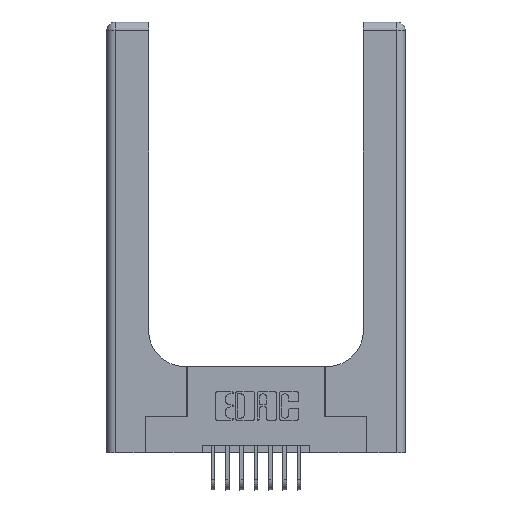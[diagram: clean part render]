
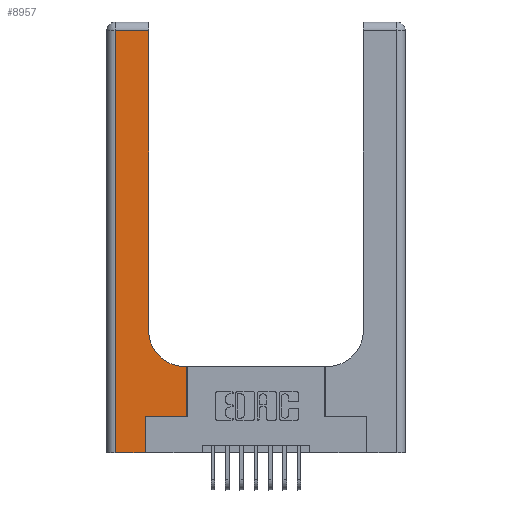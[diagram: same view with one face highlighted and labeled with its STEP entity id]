
A CAD part, top view. The second image highlights one B-rep face of the part: STEP entity #8957.
In plain terms, the highlighted planar face has unit normal (0, 0, 1).
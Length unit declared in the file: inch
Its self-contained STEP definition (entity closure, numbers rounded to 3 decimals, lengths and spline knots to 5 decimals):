
#99 = ORIENTED_EDGE ( 'NONE', *, *, #4465, .T. ) ;
#174 = LINE ( 'NONE', #6906, #6595 ) ;
#306 = AXIS2_PLACEMENT_3D ( 'NONE', #1121, #5297, #14372 ) ;
#1121 = CARTESIAN_POINT ( 'NONE',  ( 0., 3., 0.37 ) ) ;
#1159 = ORIENTED_EDGE ( 'NONE', *, *, #1406, .T. ) ;
#1214 = ORIENTED_EDGE ( 'NONE', *, *, #3346, .T. ) ;
#1329 = ORIENTED_EDGE ( 'NONE', *, *, #3376, .T. ) ;
#1394 = VERTEX_POINT ( 'NONE', #12802 ) ;
#1406 = EDGE_CURVE ( 'NONE', #1394, #3096, #4149, .T. ) ;
#1425 = VERTEX_POINT ( 'NONE', #12467 ) ;
#1510 = LINE ( 'NONE', #16889, #15101 ) ;
#1581 = ORIENTED_EDGE ( 'NONE', *, *, #5345, .T. ) ;
#1689 = VECTOR ( 'NONE', #13584, 39.37008 ) ;
#2341 = CIRCLE ( 'NONE', #14612, 0.25 ) ;
#2846 = DIRECTION ( 'NONE',  ( 0., 0., -1. ) ) ;
#3096 = VERTEX_POINT ( 'NONE', #14969 ) ;
#3267 = CARTESIAN_POINT ( 'NONE',  ( 0.5415, 0.6, 0.37 ) ) ;
#3346 = EDGE_CURVE ( 'NONE', #13283, #1394, #9100, .T. ) ;
#3376 = EDGE_CURVE ( 'NONE', #1425, #16969, #1510, .T. ) ;
#3851 = DIRECTION ( 'NONE',  ( 0., -1., 0. ) ) ;
#3909 = VERTEX_POINT ( 'NONE', #16985 ) ;
#4041 = EDGE_CURVE ( 'NONE', #3096, #5231, #174, .T. ) ;
#4146 = EDGE_CURVE ( 'NONE', #5231, #3909, #4934, .T. ) ;
#4149 = LINE ( 'NONE', #12658, #13765 ) ;
#4465 = EDGE_CURVE ( 'NONE', #16969, #13283, #8037, .T. ) ;
#4934 = LINE ( 'NONE', #12531, #15663 ) ;
#5231 = VERTEX_POINT ( 'NONE', #8025 ) ;
#5243 = ORIENTED_EDGE ( 'NONE', *, *, #4146, .T. ) ;
#5297 = DIRECTION ( 'NONE',  ( 0., 0., -1. ) ) ;
#5345 = EDGE_CURVE ( 'NONE', #3909, #15047, #5358, .T. ) ;
#5357 = DIRECTION ( 'NONE',  ( 0., 1., 0. ) ) ;
#5358 = LINE ( 'NONE', #16061, #1689 ) ;
#5701 = ORIENTED_EDGE ( 'NONE', *, *, #11182, .T. ) ;
#5800 = DIRECTION ( 'NONE',  ( -1., 0., 0. ) ) ;
#6087 = ORIENTED_EDGE ( 'NONE', *, *, #4041, .T. ) ;
#6595 = VECTOR ( 'NONE', #15938, 39.37008 ) ;
#6906 = CARTESIAN_POINT ( 'NONE',  ( 0.269, 0., 0.37 ) ) ;
#7867 = CARTESIAN_POINT ( 'NONE',  ( 0., 2.94, 0.37 ) ) ;
#8025 = CARTESIAN_POINT ( 'NONE',  ( 0.269, 0.25, 0.37 ) ) ;
#8037 = LINE ( 'NONE', #7867, #14897 ) ;
#8122 = EDGE_LOOP ( 'NONE', ( #1329, #99, #1214, #1159, #6087, #5243, #1581, #5701, #9970 ) ) ;
#8163 = LINE ( 'NONE', #9796, #14629 ) ;
#8587 = DIRECTION ( 'NONE',  ( 1., 0., 0. ) ) ;
#8628 = CARTESIAN_POINT ( 'NONE',  ( 0.2915, 2.94, 0.37 ) ) ;
#8957 = ADVANCED_FACE ( 'NONE', ( #16131 ), #11827, .F. ) ;
#9100 = LINE ( 'NONE', #13112, #15888 ) ;
#9796 = CARTESIAN_POINT ( 'NONE',  ( 0.2915, 0.6, 0.37 ) ) ;
#9944 = CARTESIAN_POINT ( 'NONE',  ( 0.06, 2.94, 0.37 ) ) ;
#9970 = ORIENTED_EDGE ( 'NONE', *, *, #16236, .T. ) ;
#10869 = CARTESIAN_POINT ( 'NONE',  ( 0.5415, 0.85, 0.37 ) ) ;
#11182 = EDGE_CURVE ( 'NONE', #15047, #13286, #8163, .T. ) ;
#11827 = PLANE ( 'NONE',  #306 ) ;
#12141 = DIRECTION ( 'NONE',  ( 1., 0., 0. ) ) ;
#12467 = CARTESIAN_POINT ( 'NONE',  ( 0.2915, 0.85, 0.37 ) ) ;
#12531 = CARTESIAN_POINT ( 'NONE',  ( 0.269, 0.25, 0.37 ) ) ;
#12572 = DIRECTION ( 'NONE',  ( 1., 0., 0. ) ) ;
#12658 = CARTESIAN_POINT ( 'NONE',  ( 0., 0., 0.37 ) ) ;
#12802 = CARTESIAN_POINT ( 'NONE',  ( 0.06, 0., 0.37 ) ) ;
#13112 = CARTESIAN_POINT ( 'NONE',  ( 0.06, 3., 0.37 ) ) ;
#13283 = VERTEX_POINT ( 'NONE', #9944 ) ;
#13286 = VERTEX_POINT ( 'NONE', #3267 ) ;
#13584 = DIRECTION ( 'NONE',  ( 0., 1., 0. ) ) ;
#13765 = VECTOR ( 'NONE', #12572, 39.37008 ) ;
#14372 = DIRECTION ( 'NONE',  ( -1., 0., 0. ) ) ;
#14612 = AXIS2_PLACEMENT_3D ( 'NONE', #10869, #2846, #12141 ) ;
#14629 = VECTOR ( 'NONE', #5800, 39.37008 ) ;
#14897 = VECTOR ( 'NONE', #16853, 39.37008 ) ;
#14969 = CARTESIAN_POINT ( 'NONE',  ( 0.269, 0., 0.37 ) ) ;
#15047 = VERTEX_POINT ( 'NONE', #16176 ) ;
#15101 = VECTOR ( 'NONE', #5357, 39.37008 ) ;
#15663 = VECTOR ( 'NONE', #8587, 39.37008 ) ;
#15888 = VECTOR ( 'NONE', #3851, 39.37008 ) ;
#15938 = DIRECTION ( 'NONE',  ( 0., 1., 0. ) ) ;
#16061 = CARTESIAN_POINT ( 'NONE',  ( 0.5585, 0.25, 0.37 ) ) ;
#16131 = FACE_OUTER_BOUND ( 'NONE', #8122, .T. ) ;
#16176 = CARTESIAN_POINT ( 'NONE',  ( 0.5585, 0.6, 0.37 ) ) ;
#16236 = EDGE_CURVE ( 'NONE', #13286, #1425, #2341, .T. ) ;
#16853 = DIRECTION ( 'NONE',  ( -1., 0., 0. ) ) ;
#16889 = CARTESIAN_POINT ( 'NONE',  ( 0.2915, 3., 0.37 ) ) ;
#16969 = VERTEX_POINT ( 'NONE', #8628 ) ;
#16985 = CARTESIAN_POINT ( 'NONE',  ( 0.5585, 0.25, 0.37 ) ) ;
